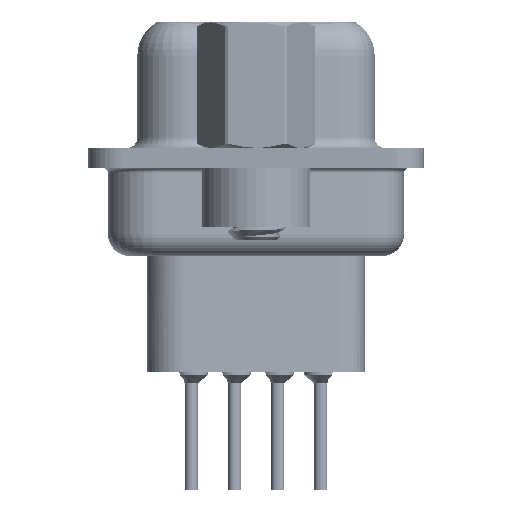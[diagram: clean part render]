
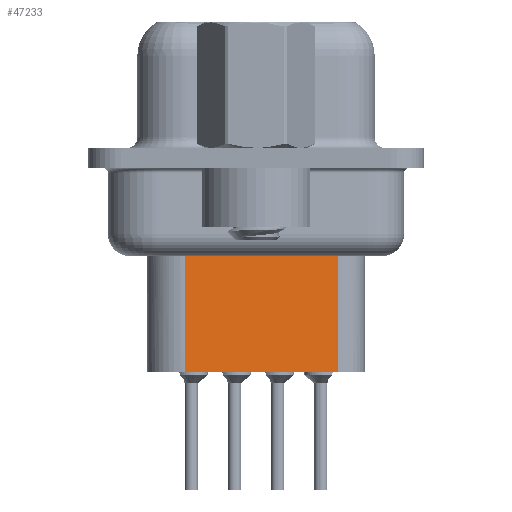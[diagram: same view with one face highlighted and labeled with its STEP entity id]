
A CAD part, left-side view. The second image highlights one B-rep face of the part: STEP entity #47233.
In plain terms, the highlighted planar face has unit normal (-0.985, -0.174, 0).
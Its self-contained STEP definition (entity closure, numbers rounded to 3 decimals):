
#1584 = CARTESIAN_POINT ( 'NONE',  ( 5.858, -3.76, -9.85 ) ) ;
#2448 = VERTEX_POINT ( 'NONE', #50327 ) ;
#3049 = EDGE_CURVE ( 'NONE', #29755, #2448, #41367, .T. ) ;
#5477 = EDGE_CURVE ( 'NONE', #58684, #2448, #40625, .T. ) ;
#6200 = CARTESIAN_POINT ( 'NONE',  ( 4.624, 3.24, -9.85 ) ) ;
#7128 = DIRECTION ( 'NONE',  ( -0.174, 0.985, 0. ) ) ;
#7495 = ORIENTED_EDGE ( 'NONE', *, *, #34489, .T. ) ;
#7514 = VERTEX_POINT ( 'NONE', #26233 ) ;
#9420 = CARTESIAN_POINT ( 'NONE',  ( 4.624, 3.24, -3.1 ) ) ;
#14206 = EDGE_CURVE ( 'NONE', #7514, #58684, #52999, .T. ) ;
#15039 = DIRECTION ( 'NONE',  ( 0., 0., -1. ) ) ;
#17712 = VECTOR ( 'NONE', #7128, 1000. ) ;
#17937 = AXIS2_PLACEMENT_3D ( 'NONE', #9420, #58732, #20145 ) ;
#20145 = DIRECTION ( 'NONE',  ( 0.174, -0.985, 0. ) ) ;
#22346 = DIRECTION ( 'NONE',  ( -0.174, 0.985, 0. ) ) ;
#25197 = FACE_OUTER_BOUND ( 'NONE', #51904, .T. ) ;
#26233 = CARTESIAN_POINT ( 'NONE',  ( 5.858, -3.76, -3.975 ) ) ;
#27132 = CARTESIAN_POINT ( 'NONE',  ( 4.624, 3.24, -3.1 ) ) ;
#28949 = CARTESIAN_POINT ( 'NONE',  ( 5.858, -3.76, -3.1 ) ) ;
#29755 = VERTEX_POINT ( 'NONE', #53421 ) ;
#32797 = DIRECTION ( 'NONE',  ( 0., 0., -1. ) ) ;
#34489 = EDGE_CURVE ( 'NONE', #7514, #29755, #51447, .T. ) ;
#40625 = LINE ( 'NONE', #6200, #17712 ) ;
#41367 = LINE ( 'NONE', #27132, #58312 ) ;
#42274 = CARTESIAN_POINT ( 'NONE',  ( 4.453, 4.209, -3.975 ) ) ;
#44171 = PLANE ( 'NONE',  #17937 ) ;
#45515 = ORIENTED_EDGE ( 'NONE', *, *, #3049, .T. ) ;
#47233 = ADVANCED_FACE ( 'NONE', ( #25197 ), #44171, .T. ) ;
#50327 = CARTESIAN_POINT ( 'NONE',  ( 4.624, 3.24, -9.85 ) ) ;
#51447 = LINE ( 'NONE', #42274, #56109 ) ;
#51904 = EDGE_LOOP ( 'NONE', ( #53870, #7495, #45515, #54622 ) ) ;
#52999 = LINE ( 'NONE', #28949, #55723 ) ;
#53421 = CARTESIAN_POINT ( 'NONE',  ( 4.624, 3.24, -3.975 ) ) ;
#53870 = ORIENTED_EDGE ( 'NONE', *, *, #14206, .F. ) ;
#54622 = ORIENTED_EDGE ( 'NONE', *, *, #5477, .F. ) ;
#55723 = VECTOR ( 'NONE', #15039, 1000. ) ;
#56109 = VECTOR ( 'NONE', #22346, 1000. ) ;
#58312 = VECTOR ( 'NONE', #32797, 1000. ) ;
#58684 = VERTEX_POINT ( 'NONE', #1584 ) ;
#58732 = DIRECTION ( 'NONE',  ( -0.985, -0.174, 0. ) ) ;
